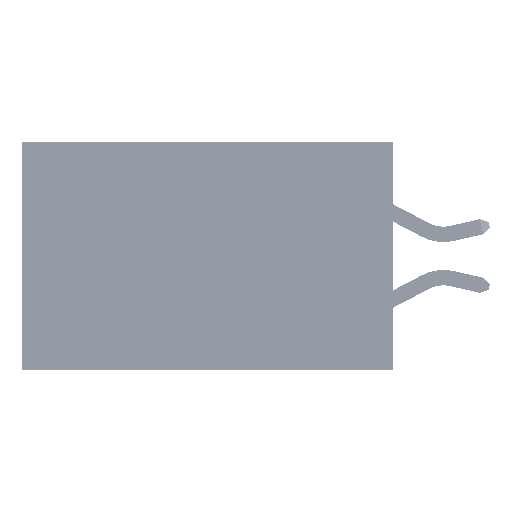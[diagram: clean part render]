
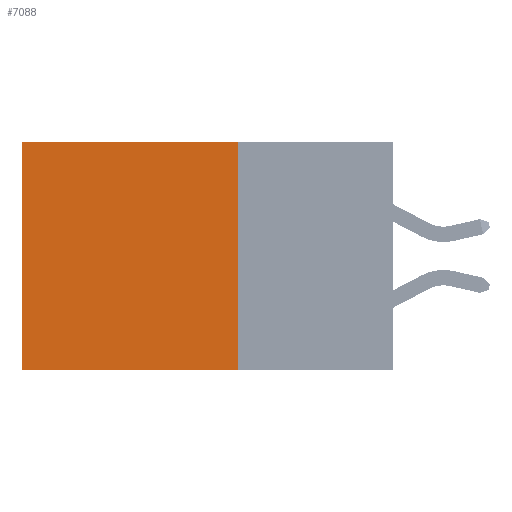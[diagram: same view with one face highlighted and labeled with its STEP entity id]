
A CAD part, left-side view. The second image highlights one B-rep face of the part: STEP entity #7088.
In plain terms, the highlighted planar face has unit normal (-1, 0, 0).
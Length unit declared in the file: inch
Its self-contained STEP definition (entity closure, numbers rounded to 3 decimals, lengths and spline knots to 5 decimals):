
#1859 = CARTESIAN_POINT ( 'NONE',  ( 0.2875, 0.25, -0.37 ) ) ;
#3787 = FACE_OUTER_BOUND ( 'NONE', #24094, .T. ) ;
#5039 = LINE ( 'NONE', #1859, #24883 ) ;
#6843 = VERTEX_POINT ( 'NONE', #10195 ) ;
#7088 = ADVANCED_FACE ( 'NONE', ( #3787 ), #15350, .F. ) ;
#8516 = EDGE_CURVE ( 'NONE', #15425, #37549, #40464, .T. ) ;
#10195 = CARTESIAN_POINT ( 'NONE',  ( 0.2875, 0.6, 0. ) ) ;
#10413 = DIRECTION ( 'NONE',  ( 0., 1., 0. ) ) ;
#11599 = ORIENTED_EDGE ( 'NONE', *, *, #13613, .T. ) ;
#12156 = VERTEX_POINT ( 'NONE', #21979 ) ;
#13613 = EDGE_CURVE ( 'NONE', #6843, #12156, #28698, .T. ) ;
#15350 = PLANE ( 'NONE',  #37784 ) ;
#15425 = VERTEX_POINT ( 'NONE', #30263 ) ;
#15761 = EDGE_CURVE ( 'NONE', #15425, #6843, #30792, .T. ) ;
#20185 = CARTESIAN_POINT ( 'NONE',  ( 0.2875, 0.6, 0. ) ) ;
#21929 = CARTESIAN_POINT ( 'NONE',  ( 0.2875, 0.25, -0.37 ) ) ;
#21979 = CARTESIAN_POINT ( 'NONE',  ( 0.2875, 0.6, -0.37 ) ) ;
#22877 = DIRECTION ( 'NONE',  ( 0., 0., -1. ) ) ;
#23932 = DIRECTION ( 'NONE',  ( 0., 0., -1. ) ) ;
#24094 = EDGE_LOOP ( 'NONE', ( #11599, #38806, #31357, #27341 ) ) ;
#24883 = VECTOR ( 'NONE', #31703, 39.37008 ) ;
#25313 = DIRECTION ( 'NONE',  ( 0., 0., -1. ) ) ;
#27341 = ORIENTED_EDGE ( 'NONE', *, *, #15761, .T. ) ;
#28698 = LINE ( 'NONE', #20185, #47220 ) ;
#28947 = CARTESIAN_POINT ( 'NONE',  ( 0.2875, 0.25, 0. ) ) ;
#29610 = VECTOR ( 'NONE', #10413, 39.37008 ) ;
#30263 = CARTESIAN_POINT ( 'NONE',  ( 0.2875, 0.25, 0. ) ) ;
#30792 = LINE ( 'NONE', #28947, #29610 ) ;
#31357 = ORIENTED_EDGE ( 'NONE', *, *, #8516, .F. ) ;
#31703 = DIRECTION ( 'NONE',  ( 0., 1., 0. ) ) ;
#33770 = CARTESIAN_POINT ( 'NONE',  ( 0.2875, 0.25, 0. ) ) ;
#37549 = VERTEX_POINT ( 'NONE', #21929 ) ;
#37784 = AXIS2_PLACEMENT_3D ( 'NONE', #33770, #45112, #22877 ) ;
#38806 = ORIENTED_EDGE ( 'NONE', *, *, #42872, .F. ) ;
#40464 = LINE ( 'NONE', #43841, #42800 ) ;
#42800 = VECTOR ( 'NONE', #25313, 39.37008 ) ;
#42872 = EDGE_CURVE ( 'NONE', #37549, #12156, #5039, .T. ) ;
#43841 = CARTESIAN_POINT ( 'NONE',  ( 0.2875, 0.25, 0. ) ) ;
#45112 = DIRECTION ( 'NONE',  ( 1., 0., 0. ) ) ;
#47220 = VECTOR ( 'NONE', #23932, 39.37008 ) ;
